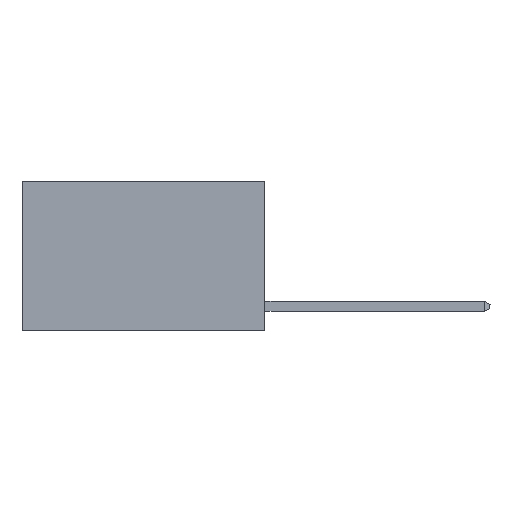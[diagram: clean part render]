
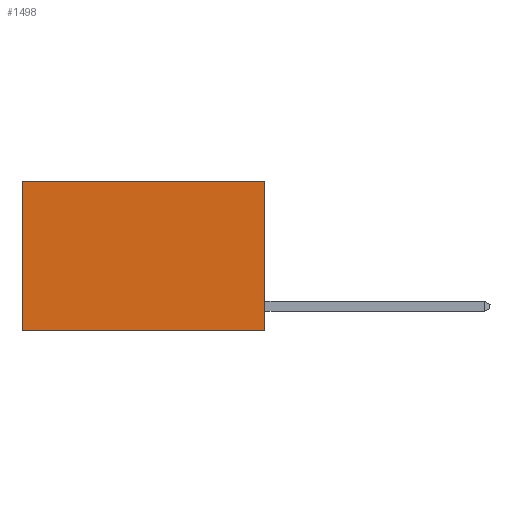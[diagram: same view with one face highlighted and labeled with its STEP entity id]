
A CAD part, left-side view. The second image highlights one B-rep face of the part: STEP entity #1498.
In plain terms, the highlighted planar face has unit normal (-1, 0, 0).
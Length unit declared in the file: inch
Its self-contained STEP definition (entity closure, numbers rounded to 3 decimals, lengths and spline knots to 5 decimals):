
#1096 = LINE ( 'NONE', #13480, #13170 ) ;
#1466 = VECTOR ( 'NONE', #2198, 39.37008 ) ;
#1498 = ADVANCED_FACE ( 'NONE', ( #6498 ), #6883, .F. ) ;
#1637 = EDGE_LOOP ( 'NONE', ( #4781, #7833, #13658, #2022 ) ) ;
#2022 = ORIENTED_EDGE ( 'NONE', *, *, #10947, .T. ) ;
#2198 = DIRECTION ( 'NONE',  ( 0., 0., -1. ) ) ;
#2803 = DIRECTION ( 'NONE',  ( 1., 0., 0. ) ) ;
#3829 = VECTOR ( 'NONE', #10473, 39.37008 ) ;
#4051 = CARTESIAN_POINT ( 'NONE',  ( 0.2625, 0., 0. ) ) ;
#4175 = VERTEX_POINT ( 'NONE', #4743 ) ;
#4743 = CARTESIAN_POINT ( 'NONE',  ( 0.2625, 0., 0. ) ) ;
#4781 = ORIENTED_EDGE ( 'NONE', *, *, #10933, .T. ) ;
#5078 = CARTESIAN_POINT ( 'NONE',  ( 0.2625, 0., -0.37 ) ) ;
#5118 = VERTEX_POINT ( 'NONE', #12470 ) ;
#5125 = DIRECTION ( 'NONE',  ( 0., 1., 0. ) ) ;
#5474 = DIRECTION ( 'NONE',  ( 0., 0., -1. ) ) ;
#5722 = DIRECTION ( 'NONE',  ( 0., 1., 0. ) ) ;
#6050 = AXIS2_PLACEMENT_3D ( 'NONE', #4051, #2803, #5474 ) ;
#6498 = FACE_OUTER_BOUND ( 'NONE', #1637, .T. ) ;
#6845 = CARTESIAN_POINT ( 'NONE',  ( 0.2625, 0.6, 0. ) ) ;
#6883 = PLANE ( 'NONE',  #6050 ) ;
#7104 = VERTEX_POINT ( 'NONE', #6845 ) ;
#7596 = VERTEX_POINT ( 'NONE', #13154 ) ;
#7833 = ORIENTED_EDGE ( 'NONE', *, *, #13346, .F. ) ;
#7982 = VECTOR ( 'NONE', #5125, 39.37008 ) ;
#8339 = LINE ( 'NONE', #5078, #7982 ) ;
#9351 = CARTESIAN_POINT ( 'NONE',  ( 0.2625, 0., 0. ) ) ;
#9907 = LINE ( 'NONE', #9351, #3829 ) ;
#10243 = CARTESIAN_POINT ( 'NONE',  ( 0.2625, 0.6, 0. ) ) ;
#10473 = DIRECTION ( 'NONE',  ( 0., 0., -1. ) ) ;
#10933 = EDGE_CURVE ( 'NONE', #7104, #5118, #13505, .T. ) ;
#10947 = EDGE_CURVE ( 'NONE', #4175, #7104, #1096, .T. ) ;
#12470 = CARTESIAN_POINT ( 'NONE',  ( 0.2625, 0.6, -0.37 ) ) ;
#12644 = EDGE_CURVE ( 'NONE', #4175, #7596, #9907, .T. ) ;
#13154 = CARTESIAN_POINT ( 'NONE',  ( 0.2625, 0., -0.37 ) ) ;
#13170 = VECTOR ( 'NONE', #5722, 39.37008 ) ;
#13346 = EDGE_CURVE ( 'NONE', #7596, #5118, #8339, .T. ) ;
#13480 = CARTESIAN_POINT ( 'NONE',  ( 0.2625, 0., 0. ) ) ;
#13505 = LINE ( 'NONE', #10243, #1466 ) ;
#13658 = ORIENTED_EDGE ( 'NONE', *, *, #12644, .F. ) ;
